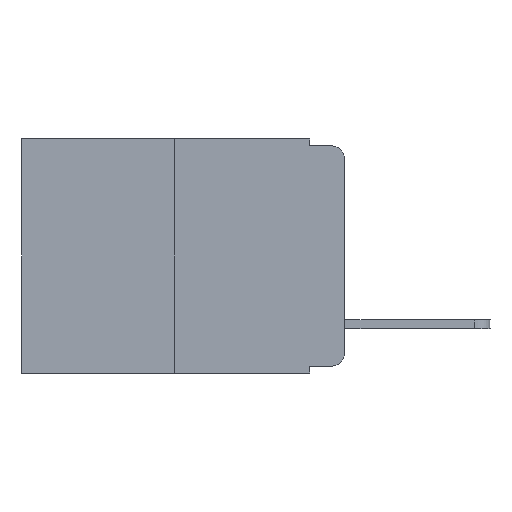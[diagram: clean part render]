
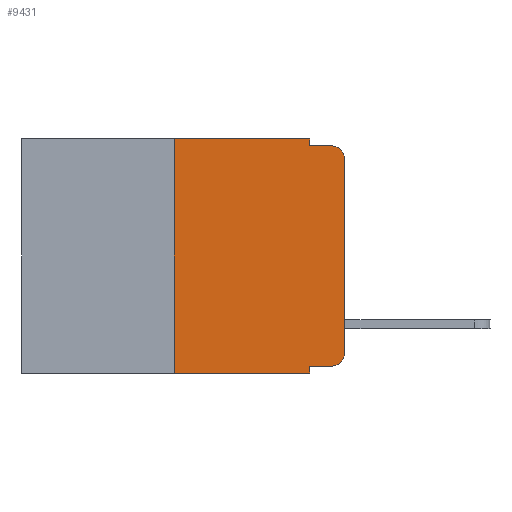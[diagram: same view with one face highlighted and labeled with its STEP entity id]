
A CAD part, left-side view. The second image highlights one B-rep face of the part: STEP entity #9431.
In plain terms, the highlighted planar face has unit normal (-1, 0, 0).
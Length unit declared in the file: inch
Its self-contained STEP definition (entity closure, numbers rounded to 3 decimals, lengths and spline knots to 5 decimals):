
#33 = VECTOR ( 'NONE', #17129, 39.37008 ) ;
#35 = AXIS2_PLACEMENT_3D ( 'NONE', #18532, #10050, #1125 ) ;
#271 = DIRECTION ( 'NONE',  ( 0., -1., 0. ) ) ;
#463 = LINE ( 'NONE', #8688, #10971 ) ;
#519 = VERTEX_POINT ( 'NONE', #17308 ) ;
#645 = DIRECTION ( 'NONE',  ( 0., -1., 0. ) ) ;
#987 = CARTESIAN_POINT ( 'NONE',  ( 0., 0., -0.03 ) ) ;
#1006 = EDGE_CURVE ( 'NONE', #5287, #1026, #463, .T. ) ;
#1026 = VERTEX_POINT ( 'NONE', #15719 ) ;
#1125 = DIRECTION ( 'NONE',  ( 0., 0., -1. ) ) ;
#1172 = LINE ( 'NONE', #8778, #8668 ) ;
#1214 = LINE ( 'NONE', #18715, #8711 ) ;
#1336 = ORIENTED_EDGE ( 'NONE', *, *, #4992, .F. ) ;
#1531 = CARTESIAN_POINT ( 'NONE',  ( 0., 0.25, -0.343 ) ) ;
#1844 = ORIENTED_EDGE ( 'NONE', *, *, #15974, .F. ) ;
#2052 = EDGE_CURVE ( 'NONE', #17851, #15094, #1172, .T. ) ;
#2188 = AXIS2_PLACEMENT_3D ( 'NONE', #2743, #12951, #4203 ) ;
#2743 = CARTESIAN_POINT ( 'NONE',  ( 0., 0.02, -0.313 ) ) ;
#2773 = VECTOR ( 'NONE', #11485, 39.37008 ) ;
#2961 = DIRECTION ( 'NONE',  ( 0., 0., 1. ) ) ;
#3002 = LINE ( 'NONE', #9637, #18375 ) ;
#3241 = LINE ( 'NONE', #7060, #33 ) ;
#3795 = CARTESIAN_POINT ( 'NONE',  ( 0., 0.02, -0.01 ) ) ;
#4052 = EDGE_CURVE ( 'NONE', #519, #16109, #4845, .T. ) ;
#4066 = VERTEX_POINT ( 'NONE', #15263 ) ;
#4203 = DIRECTION ( 'NONE',  ( 0., 0., -1. ) ) ;
#4296 = DIRECTION ( 'NONE',  ( 0., -1., 0. ) ) ;
#4845 = LINE ( 'NONE', #11025, #12196 ) ;
#4992 = EDGE_CURVE ( 'NONE', #16109, #5020, #3002, .T. ) ;
#5020 = VERTEX_POINT ( 'NONE', #3795 ) ;
#5287 = VERTEX_POINT ( 'NONE', #11704 ) ;
#6137 = CARTESIAN_POINT ( 'NONE',  ( 0., 0.473, 0. ) ) ;
#6210 = ORIENTED_EDGE ( 'NONE', *, *, #2052, .F. ) ;
#7020 = EDGE_CURVE ( 'NONE', #10377, #5020, #8794, .T. ) ;
#7060 = CARTESIAN_POINT ( 'NONE',  ( 0., 0.473, 0. ) ) ;
#7199 = ORIENTED_EDGE ( 'NONE', *, *, #17979, .T. ) ;
#7697 = DIRECTION ( 'NONE',  ( 0., 0., -1. ) ) ;
#7954 = DIRECTION ( 'NONE',  ( 0., 0., -1. ) ) ;
#8035 = EDGE_CURVE ( 'NONE', #17145, #10377, #14366, .T. ) ;
#8668 = VECTOR ( 'NONE', #2961, 39.37008 ) ;
#8688 = CARTESIAN_POINT ( 'NONE',  ( 0., 0.051, 0. ) ) ;
#8711 = VECTOR ( 'NONE', #4296, 39.37008 ) ;
#8778 = CARTESIAN_POINT ( 'NONE',  ( 0., 0.25, 0. ) ) ;
#8794 = CIRCLE ( 'NONE', #35, 0.02 ) ;
#8832 = ORIENTED_EDGE ( 'NONE', *, *, #7020, .T. ) ;
#9431 = ADVANCED_FACE ( 'NONE', ( #16320 ), #13378, .F. ) ;
#9637 = CARTESIAN_POINT ( 'NONE',  ( 0., 0.051, -0.01 ) ) ;
#9899 = EDGE_CURVE ( 'NONE', #17851, #1026, #1214, .T. ) ;
#10050 = DIRECTION ( 'NONE',  ( -1., 0., 0. ) ) ;
#10060 = CARTESIAN_POINT ( 'NONE',  ( 0., 0., 0. ) ) ;
#10113 = EDGE_LOOP ( 'NONE', ( #15966, #8832, #1336, #16874, #1844, #6210, #17757, #18206, #7199, #11529 ) ) ;
#10377 = VERTEX_POINT ( 'NONE', #987 ) ;
#10971 = VECTOR ( 'NONE', #7954, 39.37008 ) ;
#11025 = CARTESIAN_POINT ( 'NONE',  ( 0., 0.051, 0. ) ) ;
#11150 = VECTOR ( 'NONE', #271, 39.37008 ) ;
#11485 = DIRECTION ( 'NONE',  ( 0., 0., 1. ) ) ;
#11529 = ORIENTED_EDGE ( 'NONE', *, *, #17033, .T. ) ;
#11657 = CIRCLE ( 'NONE', #2188, 0.02 ) ;
#11704 = CARTESIAN_POINT ( 'NONE',  ( 0., 0.051, -0.333 ) ) ;
#11910 = CARTESIAN_POINT ( 'NONE',  ( 0., 0.051, -0.01 ) ) ;
#12196 = VECTOR ( 'NONE', #14458, 39.37008 ) ;
#12951 = DIRECTION ( 'NONE',  ( -1., 0., 0. ) ) ;
#13378 = PLANE ( 'NONE',  #16214 ) ;
#13596 = CARTESIAN_POINT ( 'NONE',  ( 0., 0.051, -0.333 ) ) ;
#14366 = LINE ( 'NONE', #10060, #2773 ) ;
#14458 = DIRECTION ( 'NONE',  ( 0., 0., -1. ) ) ;
#14467 = LINE ( 'NONE', #13596, #11150 ) ;
#14554 = CARTESIAN_POINT ( 'NONE',  ( 0., 0., -0.313 ) ) ;
#15094 = VERTEX_POINT ( 'NONE', #16208 ) ;
#15263 = CARTESIAN_POINT ( 'NONE',  ( 0., 0.02, -0.333 ) ) ;
#15719 = CARTESIAN_POINT ( 'NONE',  ( 0., 0.051, -0.343 ) ) ;
#15966 = ORIENTED_EDGE ( 'NONE', *, *, #8035, .T. ) ;
#15974 = EDGE_CURVE ( 'NONE', #15094, #519, #3241, .T. ) ;
#16109 = VERTEX_POINT ( 'NONE', #11910 ) ;
#16208 = CARTESIAN_POINT ( 'NONE',  ( 0., 0.25, 0. ) ) ;
#16214 = AXIS2_PLACEMENT_3D ( 'NONE', #6137, #16292, #7697 ) ;
#16292 = DIRECTION ( 'NONE',  ( 1., 0., 0. ) ) ;
#16320 = FACE_OUTER_BOUND ( 'NONE', #10113, .T. ) ;
#16874 = ORIENTED_EDGE ( 'NONE', *, *, #4052, .F. ) ;
#17033 = EDGE_CURVE ( 'NONE', #4066, #17145, #11657, .T. ) ;
#17129 = DIRECTION ( 'NONE',  ( 0., -1., 0. ) ) ;
#17145 = VERTEX_POINT ( 'NONE', #14554 ) ;
#17308 = CARTESIAN_POINT ( 'NONE',  ( 0., 0.051, 0. ) ) ;
#17757 = ORIENTED_EDGE ( 'NONE', *, *, #9899, .T. ) ;
#17851 = VERTEX_POINT ( 'NONE', #1531 ) ;
#17979 = EDGE_CURVE ( 'NONE', #5287, #4066, #14467, .T. ) ;
#18206 = ORIENTED_EDGE ( 'NONE', *, *, #1006, .F. ) ;
#18375 = VECTOR ( 'NONE', #645, 39.37008 ) ;
#18532 = CARTESIAN_POINT ( 'NONE',  ( 0., 0.02, -0.03 ) ) ;
#18715 = CARTESIAN_POINT ( 'NONE',  ( 0., 0.473, -0.343 ) ) ;
